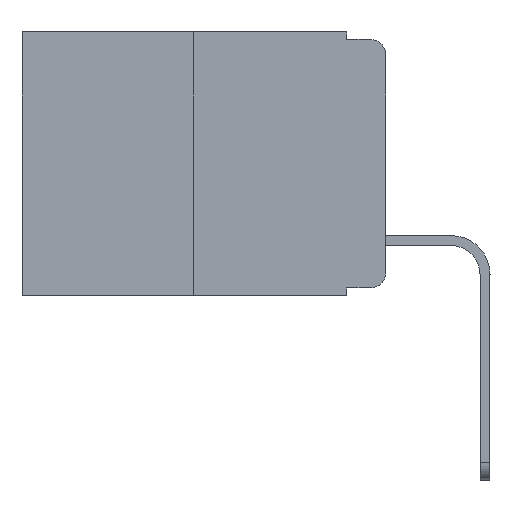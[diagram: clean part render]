
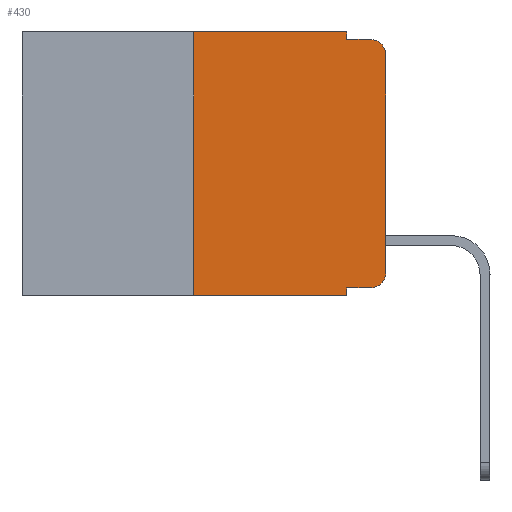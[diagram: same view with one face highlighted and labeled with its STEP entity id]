
A CAD part, left-side view. The second image highlights one B-rep face of the part: STEP entity #430.
In plain terms, the highlighted planar face has unit normal (-1, 0, 0).
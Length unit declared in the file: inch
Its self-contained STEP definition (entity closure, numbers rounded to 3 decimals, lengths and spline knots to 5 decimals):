
#38 = LINE ( 'NONE', #1175, #913 ) ;
#173 = EDGE_CURVE ( 'NONE', #6823, #3009, #2555, .T. ) ;
#430 = ADVANCED_FACE ( 'NONE', ( #3180 ), #10327, .F. ) ;
#489 = ORIENTED_EDGE ( 'NONE', *, *, #1751, .F. ) ;
#833 = AXIS2_PLACEMENT_3D ( 'NONE', #2171, #2207, #4657 ) ;
#913 = VECTOR ( 'NONE', #3730, 39.37008 ) ;
#1175 = CARTESIAN_POINT ( 'NONE',  ( 0., 0.473, -0.343 ) ) ;
#1233 = CARTESIAN_POINT ( 'NONE',  ( 0., 0., 0. ) ) ;
#1395 = VECTOR ( 'NONE', #2042, 39.37008 ) ;
#1440 = LINE ( 'NONE', #9052, #6975 ) ;
#1466 = VECTOR ( 'NONE', #6469, 39.37008 ) ;
#1552 = EDGE_CURVE ( 'NONE', #3275, #5733, #3522, .T. ) ;
#1751 = EDGE_CURVE ( 'NONE', #8942, #5150, #5272, .T. ) ;
#2042 = DIRECTION ( 'NONE',  ( 0., -1., 0. ) ) ;
#2171 = CARTESIAN_POINT ( 'NONE',  ( 0., 0.473, 0. ) ) ;
#2207 = DIRECTION ( 'NONE',  ( 1., 0., 0. ) ) ;
#2324 = ORIENTED_EDGE ( 'NONE', *, *, #3717, .F. ) ;
#2555 = LINE ( 'NONE', #8434, #1395 ) ;
#2620 = ORIENTED_EDGE ( 'NONE', *, *, #10381, .T. ) ;
#2653 = VERTEX_POINT ( 'NONE', #8087 ) ;
#2779 = EDGE_CURVE ( 'NONE', #2653, #9812, #6872, .T. ) ;
#2780 = VERTEX_POINT ( 'NONE', #4068 ) ;
#3009 = VERTEX_POINT ( 'NONE', #9242 ) ;
#3163 = ORIENTED_EDGE ( 'NONE', *, *, #9990, .F. ) ;
#3180 = FACE_OUTER_BOUND ( 'NONE', #6728, .T. ) ;
#3275 = VERTEX_POINT ( 'NONE', #8753 ) ;
#3522 = LINE ( 'NONE', #1233, #6516 ) ;
#3592 = DIRECTION ( 'NONE',  ( 0., 0., 1. ) ) ;
#3658 = CIRCLE ( 'NONE', #4969, 0.02 ) ;
#3672 = EDGE_CURVE ( 'NONE', #9812, #8942, #1440, .T. ) ;
#3717 = EDGE_CURVE ( 'NONE', #5150, #6873, #8500, .T. ) ;
#3730 = DIRECTION ( 'NONE',  ( 0., -1., 0. ) ) ;
#3776 = LINE ( 'NONE', #5416, #7891 ) ;
#3922 = ORIENTED_EDGE ( 'NONE', *, *, #7058, .T. ) ;
#4068 = CARTESIAN_POINT ( 'NONE',  ( 0., 0.051, -0.343 ) ) ;
#4109 = DIRECTION ( 'NONE',  ( 0., -1., 0. ) ) ;
#4111 = DIRECTION ( 'NONE',  ( 0., 0., -1. ) ) ;
#4124 = CARTESIAN_POINT ( 'NONE',  ( 0., 0.051, -0.01 ) ) ;
#4642 = VECTOR ( 'NONE', #9757, 39.37008 ) ;
#4657 = DIRECTION ( 'NONE',  ( 0., 0., -1. ) ) ;
#4861 = ORIENTED_EDGE ( 'NONE', *, *, #3672, .F. ) ;
#4914 = ORIENTED_EDGE ( 'NONE', *, *, #1552, .T. ) ;
#4969 = AXIS2_PLACEMENT_3D ( 'NONE', #6909, #6102, #10220 ) ;
#5150 = VERTEX_POINT ( 'NONE', #4124 ) ;
#5272 = LINE ( 'NONE', #6907, #4642 ) ;
#5416 = CARTESIAN_POINT ( 'NONE',  ( 0., 0.051, 0. ) ) ;
#5613 = CARTESIAN_POINT ( 'NONE',  ( 0., 0.25, 0. ) ) ;
#5733 = VERTEX_POINT ( 'NONE', #8874 ) ;
#5905 = ORIENTED_EDGE ( 'NONE', *, *, #7543, .T. ) ;
#6097 = AXIS2_PLACEMENT_3D ( 'NONE', #6479, #8203, #4111 ) ;
#6102 = DIRECTION ( 'NONE',  ( -1., 0., 0. ) ) ;
#6392 = CIRCLE ( 'NONE', #6097, 0.02 ) ;
#6469 = DIRECTION ( 'NONE',  ( 0., 0., 1. ) ) ;
#6479 = CARTESIAN_POINT ( 'NONE',  ( 0., 0.02, -0.313 ) ) ;
#6516 = VECTOR ( 'NONE', #3592, 39.37008 ) ;
#6728 = EDGE_LOOP ( 'NONE', ( #4914, #3922, #2324, #489, #4861, #9307, #5905, #3163, #8940, #2620 ) ) ;
#6823 = VERTEX_POINT ( 'NONE', #8192 ) ;
#6848 = VECTOR ( 'NONE', #9748, 39.37008 ) ;
#6872 = LINE ( 'NONE', #8050, #1466 ) ;
#6873 = VERTEX_POINT ( 'NONE', #9276 ) ;
#6907 = CARTESIAN_POINT ( 'NONE',  ( 0., 0.051, 0. ) ) ;
#6909 = CARTESIAN_POINT ( 'NONE',  ( 0., 0.02, -0.03 ) ) ;
#6975 = VECTOR ( 'NONE', #4109, 39.37008 ) ;
#7058 = EDGE_CURVE ( 'NONE', #5733, #6873, #3658, .T. ) ;
#7543 = EDGE_CURVE ( 'NONE', #2653, #2780, #38, .T. ) ;
#7781 = DIRECTION ( 'NONE',  ( 0., 0., -1. ) ) ;
#7891 = VECTOR ( 'NONE', #7781, 39.37008 ) ;
#8050 = CARTESIAN_POINT ( 'NONE',  ( 0., 0.25, 0. ) ) ;
#8087 = CARTESIAN_POINT ( 'NONE',  ( 0., 0.25, -0.343 ) ) ;
#8164 = CARTESIAN_POINT ( 'NONE',  ( 0., 0.051, -0.01 ) ) ;
#8192 = CARTESIAN_POINT ( 'NONE',  ( 0., 0.051, -0.333 ) ) ;
#8203 = DIRECTION ( 'NONE',  ( -1., 0., 0. ) ) ;
#8434 = CARTESIAN_POINT ( 'NONE',  ( 0., 0.051, -0.333 ) ) ;
#8500 = LINE ( 'NONE', #8164, #6848 ) ;
#8753 = CARTESIAN_POINT ( 'NONE',  ( 0., 0., -0.313 ) ) ;
#8874 = CARTESIAN_POINT ( 'NONE',  ( 0., 0., -0.03 ) ) ;
#8940 = ORIENTED_EDGE ( 'NONE', *, *, #173, .T. ) ;
#8942 = VERTEX_POINT ( 'NONE', #9579 ) ;
#9052 = CARTESIAN_POINT ( 'NONE',  ( 0., 0.473, 0. ) ) ;
#9242 = CARTESIAN_POINT ( 'NONE',  ( 0., 0.02, -0.333 ) ) ;
#9276 = CARTESIAN_POINT ( 'NONE',  ( 0., 0.02, -0.01 ) ) ;
#9307 = ORIENTED_EDGE ( 'NONE', *, *, #2779, .F. ) ;
#9579 = CARTESIAN_POINT ( 'NONE',  ( 0., 0.051, 0. ) ) ;
#9748 = DIRECTION ( 'NONE',  ( 0., -1., 0. ) ) ;
#9757 = DIRECTION ( 'NONE',  ( 0., 0., -1. ) ) ;
#9812 = VERTEX_POINT ( 'NONE', #5613 ) ;
#9990 = EDGE_CURVE ( 'NONE', #6823, #2780, #3776, .T. ) ;
#10220 = DIRECTION ( 'NONE',  ( 0., 0., -1. ) ) ;
#10327 = PLANE ( 'NONE',  #833 ) ;
#10381 = EDGE_CURVE ( 'NONE', #3009, #3275, #6392, .T. ) ;
